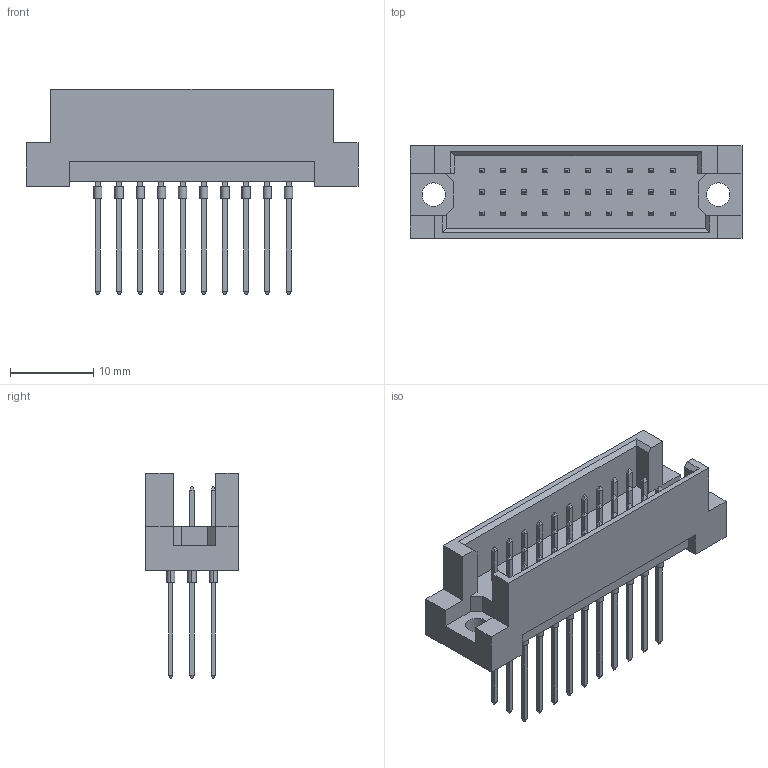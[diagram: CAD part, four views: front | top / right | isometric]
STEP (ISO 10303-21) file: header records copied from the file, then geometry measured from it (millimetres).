
FILE_DESCRIPTION (( 'STEP AP203' ), '1' );
FILE_NAME ('493-130-280-311.STEP', '2019-11-11T20:00:11', ( '' ), ( '' ), 'SwSTEP 2.0', 'SolidWorks 2020', '' );
FILE_SCHEMA (( 'CONFIG_CONTROL_DESIGN' ));
Length unit declared in the file: millimetre
Products named in the file (3): 493-130-280-311; 493-290_80; 493 Part_30
Assembly tree (31 placements, depth 2):
  493-130-280-311
    493 Part_30
    493-290_80  x30
Bounding box: 39.8 x 11.1 x 24.6 mm (x, y, z)
Volume: 2598.3 mm3; surface area: 4315.5 mm2
Topology: 31 solids, 31 shells, 832 faces, 1886 edges, 1176 vertices
Faces by surface type: plane 768, cylinder 64
Entity records: 7533 total; most frequent: CARTESIAN_POINT 1144, ORIENTED_EDGE 1104, DIRECTION 1020, EDGE_CURVE 552, VECTOR 540, LINE 540, VERTEX_POINT 364, EDGE_LOOP 260
